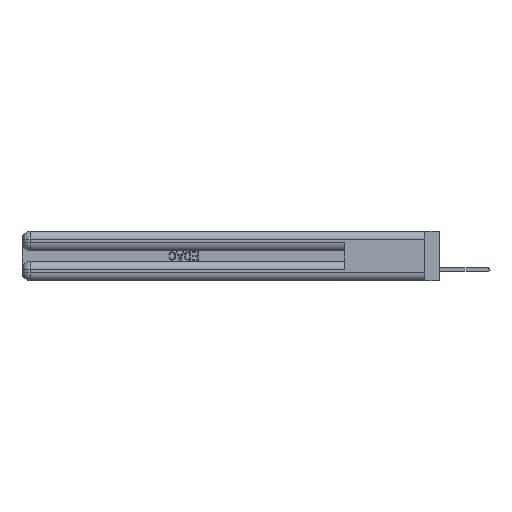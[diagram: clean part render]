
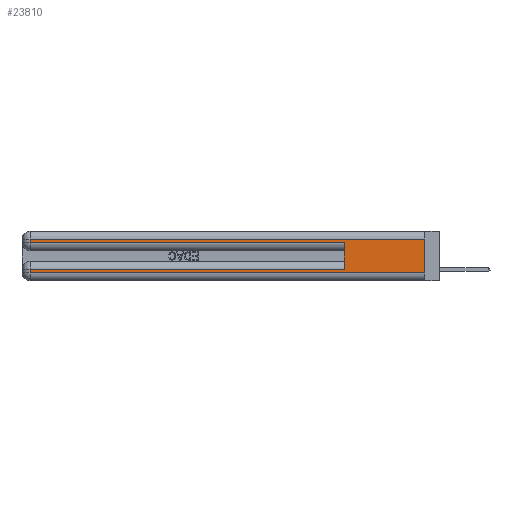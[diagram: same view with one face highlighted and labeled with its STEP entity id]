
A CAD part, left-side view. The second image highlights one B-rep face of the part: STEP entity #23810.
In plain terms, the highlighted planar face has unit normal (-1, 0, 0).
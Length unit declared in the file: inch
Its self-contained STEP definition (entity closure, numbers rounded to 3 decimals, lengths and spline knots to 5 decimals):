
#21 = ORIENTED_EDGE ( 'NONE', *, *, #41189, .T. ) ;
#1261 = EDGE_CURVE ( 'NONE', #18376, #27654, #34816, .T. ) ;
#1569 = VERTEX_POINT ( 'NONE', #27406 ) ;
#2114 = AXIS2_PLACEMENT_3D ( 'NONE', #22919, #15471, #34114 ) ;
#2606 = CARTESIAN_POINT ( 'NONE',  ( 0., 0., 0.31 ) ) ;
#3909 = DIRECTION ( 'NONE',  ( 0., 0., -1. ) ) ;
#6104 = EDGE_CURVE ( 'NONE', #47654, #41833, #7716, .T. ) ;
#6759 = ORIENTED_EDGE ( 'NONE', *, *, #1261, .T. ) ;
#7095 = CARTESIAN_POINT ( 'NONE',  ( 0., 0.6, 0.285 ) ) ;
#7716 = LINE ( 'NONE', #40568, #36172 ) ;
#7920 = ORIENTED_EDGE ( 'NONE', *, *, #13517, .T. ) ;
#8193 = CARTESIAN_POINT ( 'NONE',  ( 0., 2.94, 0.085 ) ) ;
#8289 = LINE ( 'NONE', #24720, #9506 ) ;
#9506 = VECTOR ( 'NONE', #36195, 39.37008 ) ;
#11823 = CARTESIAN_POINT ( 'NONE',  ( 0., 0., 0.06 ) ) ;
#13211 = EDGE_CURVE ( 'NONE', #18843, #18376, #29678, .T. ) ;
#13448 = VECTOR ( 'NONE', #28369, 39.37008 ) ;
#13517 = EDGE_CURVE ( 'NONE', #27654, #28087, #41778, .T. ) ;
#14665 = CARTESIAN_POINT ( 'NONE',  ( 0., 2.94, 0.37 ) ) ;
#15471 = DIRECTION ( 'NONE',  ( 1., 0., 0. ) ) ;
#16168 = ORIENTED_EDGE ( 'NONE', *, *, #18289, .F. ) ;
#18289 = EDGE_CURVE ( 'NONE', #18843, #41833, #45064, .T. ) ;
#18307 = DIRECTION ( 'NONE',  ( 0., 1., 0. ) ) ;
#18376 = VERTEX_POINT ( 'NONE', #8193 ) ;
#18843 = VERTEX_POINT ( 'NONE', #23452 ) ;
#19558 = LINE ( 'NONE', #44595, #47508 ) ;
#20147 = VECTOR ( 'NONE', #25633, 39.37008 ) ;
#21251 = FACE_OUTER_BOUND ( 'NONE', #47029, .T. ) ;
#22286 = VECTOR ( 'NONE', #18307, 39.37008 ) ;
#22597 = EDGE_CURVE ( 'NONE', #1569, #47654, #19558, .T. ) ;
#22792 = CARTESIAN_POINT ( 'NONE',  ( 0., 0., 0.085 ) ) ;
#22901 = VERTEX_POINT ( 'NONE', #41938 ) ;
#22919 = CARTESIAN_POINT ( 'NONE',  ( 0., 0., 0.37 ) ) ;
#22945 = DIRECTION ( 'NONE',  ( 0., 1., 0. ) ) ;
#23452 = CARTESIAN_POINT ( 'NONE',  ( 0., 0.6, 0.085 ) ) ;
#23810 = ADVANCED_FACE ( 'NONE', ( #21251 ), #30215, .F. ) ;
#24720 = CARTESIAN_POINT ( 'NONE',  ( 0., 0., 0.37 ) ) ;
#25633 = DIRECTION ( 'NONE',  ( 0., 0., 1. ) ) ;
#25864 = DIRECTION ( 'NONE',  ( 0., -1., 0. ) ) ;
#27406 = CARTESIAN_POINT ( 'NONE',  ( 0., 2.94, 0.31 ) ) ;
#27654 = VERTEX_POINT ( 'NONE', #44362 ) ;
#28087 = VERTEX_POINT ( 'NONE', #11823 ) ;
#28369 = DIRECTION ( 'NONE',  ( 0., -1., 0. ) ) ;
#29038 = VECTOR ( 'NONE', #44886, 39.37008 ) ;
#29678 = LINE ( 'NONE', #22792, #40096 ) ;
#30215 = PLANE ( 'NONE',  #2114 ) ;
#31213 = ORIENTED_EDGE ( 'NONE', *, *, #22597, .T. ) ;
#32719 = CARTESIAN_POINT ( 'NONE',  ( 0., 0., 0.06 ) ) ;
#32919 = CARTESIAN_POINT ( 'NONE',  ( 0., 0.6, 0.145 ) ) ;
#34114 = DIRECTION ( 'NONE',  ( 0., 0., -1. ) ) ;
#34816 = LINE ( 'NONE', #14665, #29038 ) ;
#36172 = VECTOR ( 'NONE', #25864, 39.37008 ) ;
#36195 = DIRECTION ( 'NONE',  ( 0., 0., -1. ) ) ;
#36834 = EDGE_CURVE ( 'NONE', #22901, #28087, #8289, .T. ) ;
#40096 = VECTOR ( 'NONE', #22945, 39.37008 ) ;
#40568 = CARTESIAN_POINT ( 'NONE',  ( 0., 0., 0.285 ) ) ;
#41189 = EDGE_CURVE ( 'NONE', #22901, #1569, #44875, .T. ) ;
#41778 = LINE ( 'NONE', #32719, #13448 ) ;
#41784 = ORIENTED_EDGE ( 'NONE', *, *, #6104, .T. ) ;
#41833 = VERTEX_POINT ( 'NONE', #7095 ) ;
#41938 = CARTESIAN_POINT ( 'NONE',  ( 0., 0., 0.31 ) ) ;
#44320 = ORIENTED_EDGE ( 'NONE', *, *, #36834, .F. ) ;
#44327 = ORIENTED_EDGE ( 'NONE', *, *, #13211, .T. ) ;
#44362 = CARTESIAN_POINT ( 'NONE',  ( 0., 2.94, 0.06 ) ) ;
#44595 = CARTESIAN_POINT ( 'NONE',  ( 0., 2.94, 0.37 ) ) ;
#44875 = LINE ( 'NONE', #2606, #22286 ) ;
#44886 = DIRECTION ( 'NONE',  ( 0., 0., -1. ) ) ;
#45064 = LINE ( 'NONE', #32919, #20147 ) ;
#45519 = CARTESIAN_POINT ( 'NONE',  ( 0., 2.94, 0.285 ) ) ;
#47029 = EDGE_LOOP ( 'NONE', ( #44320, #21, #31213, #41784, #16168, #44327, #6759, #7920 ) ) ;
#47508 = VECTOR ( 'NONE', #3909, 39.37008 ) ;
#47654 = VERTEX_POINT ( 'NONE', #45519 ) ;
